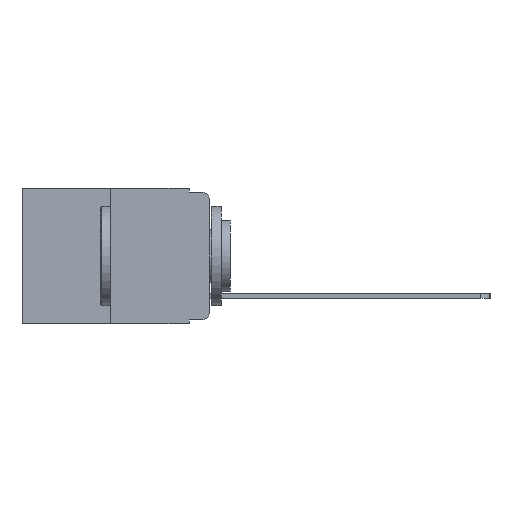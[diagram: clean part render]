
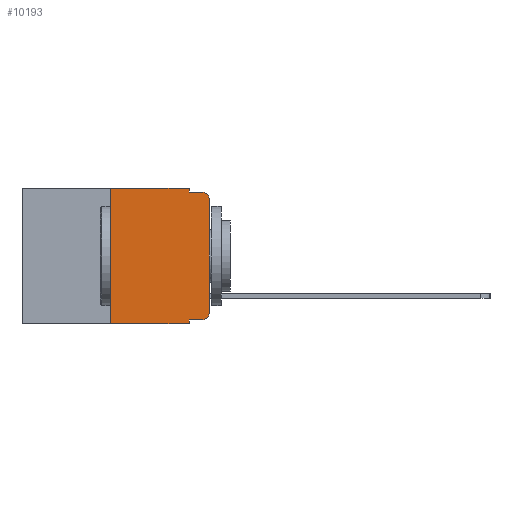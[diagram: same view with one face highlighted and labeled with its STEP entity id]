
A CAD part, left-side view. The second image highlights one B-rep face of the part: STEP entity #10193.
In plain terms, the highlighted planar face has unit normal (-1, 0, 0).
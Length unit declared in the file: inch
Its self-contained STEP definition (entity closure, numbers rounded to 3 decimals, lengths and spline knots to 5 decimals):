
#89 = ORIENTED_EDGE ( 'NONE', *, *, #8027, .F. ) ;
#531 = CARTESIAN_POINT ( 'NONE',  ( 0., 0.051, 0. ) ) ;
#598 = CARTESIAN_POINT ( 'NONE',  ( 0., 0.02, -0.313 ) ) ;
#907 = DIRECTION ( 'NONE',  ( -1., 0., 0. ) ) ;
#2142 = CARTESIAN_POINT ( 'NONE',  ( 0., 0.25, -0.343 ) ) ;
#2165 = LINE ( 'NONE', #4714, #6062 ) ;
#2266 = DIRECTION ( 'NONE',  ( 0., 0., -1. ) ) ;
#2334 = PLANE ( 'NONE',  #13816 ) ;
#2394 = VERTEX_POINT ( 'NONE', #8580 ) ;
#2579 = EDGE_CURVE ( 'NONE', #20101, #2394, #11732, .T. ) ;
#2890 = VECTOR ( 'NONE', #3605, 39.37008 ) ;
#3300 = VECTOR ( 'NONE', #14741, 39.37008 ) ;
#3605 = DIRECTION ( 'NONE',  ( 0., 0., 1. ) ) ;
#3825 = ORIENTED_EDGE ( 'NONE', *, *, #9303, .T. ) ;
#3984 = CARTESIAN_POINT ( 'NONE',  ( 0., 0.473, 0. ) ) ;
#3988 = DIRECTION ( 'NONE',  ( 0., -1., 0. ) ) ;
#3998 = DIRECTION ( 'NONE',  ( 0., 0., 1. ) ) ;
#4028 = CARTESIAN_POINT ( 'NONE',  ( 0., 0., 0. ) ) ;
#4349 = EDGE_CURVE ( 'NONE', #21163, #10808, #13995, .T. ) ;
#4439 = VECTOR ( 'NONE', #20440, 39.37008 ) ;
#4528 = DIRECTION ( 'NONE',  ( 0., -1., 0. ) ) ;
#4602 = CARTESIAN_POINT ( 'NONE',  ( 0., 0.02, -0.333 ) ) ;
#4701 = CARTESIAN_POINT ( 'NONE',  ( 0., 0., -0.03 ) ) ;
#4714 = CARTESIAN_POINT ( 'NONE',  ( 0., 0.473, -0.343 ) ) ;
#4720 = ORIENTED_EDGE ( 'NONE', *, *, #2579, .F. ) ;
#4852 = CARTESIAN_POINT ( 'NONE',  ( 0., 0.473, 0. ) ) ;
#4913 = VECTOR ( 'NONE', #3998, 39.37008 ) ;
#5105 = AXIS2_PLACEMENT_3D ( 'NONE', #598, #12107, #2266 ) ;
#5273 = CARTESIAN_POINT ( 'NONE',  ( 0., 0.25, 0. ) ) ;
#5487 = ORIENTED_EDGE ( 'NONE', *, *, #19863, .F. ) ;
#5658 = DIRECTION ( 'NONE',  ( 0., 0., -1. ) ) ;
#5970 = CIRCLE ( 'NONE', #10265, 0.02 ) ;
#6062 = VECTOR ( 'NONE', #21252, 39.37008 ) ;
#6257 = EDGE_CURVE ( 'NONE', #10003, #12196, #18077, .T. ) ;
#6425 = VERTEX_POINT ( 'NONE', #2142 ) ;
#6624 = EDGE_CURVE ( 'NONE', #12196, #10808, #5970, .T. ) ;
#6947 = VERTEX_POINT ( 'NONE', #4602 ) ;
#7085 = EDGE_LOOP ( 'NONE', ( #21006, #7484, #9443, #5487, #10631, #89, #20883, #4720, #18864, #3825 ) ) ;
#7484 = ORIENTED_EDGE ( 'NONE', *, *, #6624, .T. ) ;
#8027 = EDGE_CURVE ( 'NONE', #6425, #20708, #11605, .T. ) ;
#8580 = CARTESIAN_POINT ( 'NONE',  ( 0., 0.051, -0.343 ) ) ;
#8856 = CARTESIAN_POINT ( 'NONE',  ( 0., 0.051, 0. ) ) ;
#8939 = CARTESIAN_POINT ( 'NONE',  ( 0., 0.051, -0.333 ) ) ;
#9303 = EDGE_CURVE ( 'NONE', #6947, #10003, #19857, .T. ) ;
#9443 = ORIENTED_EDGE ( 'NONE', *, *, #4349, .F. ) ;
#9582 = VECTOR ( 'NONE', #4528, 39.37008 ) ;
#10003 = VERTEX_POINT ( 'NONE', #18994 ) ;
#10193 = ADVANCED_FACE ( 'NONE', ( #15419 ), #2334, .F. ) ;
#10265 = AXIS2_PLACEMENT_3D ( 'NONE', #20912, #907, #18419 ) ;
#10631 = ORIENTED_EDGE ( 'NONE', *, *, #13987, .F. ) ;
#10808 = VERTEX_POINT ( 'NONE', #19141 ) ;
#11506 = LINE ( 'NONE', #4852, #3300 ) ;
#11605 = LINE ( 'NONE', #5273, #2890 ) ;
#11732 = LINE ( 'NONE', #531, #16182 ) ;
#11941 = EDGE_CURVE ( 'NONE', #20101, #6947, #20548, .T. ) ;
#12107 = DIRECTION ( 'NONE',  ( -1., 0., 0. ) ) ;
#12196 = VERTEX_POINT ( 'NONE', #4701 ) ;
#13816 = AXIS2_PLACEMENT_3D ( 'NONE', #3984, #15544, #5658 ) ;
#13987 = EDGE_CURVE ( 'NONE', #20708, #14895, #11506, .T. ) ;
#13995 = LINE ( 'NONE', #14577, #9582 ) ;
#14577 = CARTESIAN_POINT ( 'NONE',  ( 0., 0.051, -0.01 ) ) ;
#14741 = DIRECTION ( 'NONE',  ( 0., -1., 0. ) ) ;
#14895 = VERTEX_POINT ( 'NONE', #20453 ) ;
#15419 = FACE_OUTER_BOUND ( 'NONE', #7085, .T. ) ;
#15544 = DIRECTION ( 'NONE',  ( 1., 0., 0. ) ) ;
#16167 = VECTOR ( 'NONE', #3988, 39.37008 ) ;
#16182 = VECTOR ( 'NONE', #18369, 39.37008 ) ;
#16317 = EDGE_CURVE ( 'NONE', #6425, #2394, #2165, .T. ) ;
#17075 = LINE ( 'NONE', #8856, #4439 ) ;
#17759 = CARTESIAN_POINT ( 'NONE',  ( 0., 0.051, -0.333 ) ) ;
#18077 = LINE ( 'NONE', #4028, #4913 ) ;
#18369 = DIRECTION ( 'NONE',  ( 0., 0., -1. ) ) ;
#18419 = DIRECTION ( 'NONE',  ( 0., 0., -1. ) ) ;
#18864 = ORIENTED_EDGE ( 'NONE', *, *, #11941, .T. ) ;
#18994 = CARTESIAN_POINT ( 'NONE',  ( 0., 0., -0.313 ) ) ;
#19141 = CARTESIAN_POINT ( 'NONE',  ( 0., 0.02, -0.01 ) ) ;
#19857 = CIRCLE ( 'NONE', #5105, 0.02 ) ;
#19863 = EDGE_CURVE ( 'NONE', #14895, #21163, #17075, .T. ) ;
#19869 = CARTESIAN_POINT ( 'NONE',  ( 0., 0.25, 0. ) ) ;
#20101 = VERTEX_POINT ( 'NONE', #17759 ) ;
#20440 = DIRECTION ( 'NONE',  ( 0., 0., -1. ) ) ;
#20453 = CARTESIAN_POINT ( 'NONE',  ( 0., 0.051, 0. ) ) ;
#20548 = LINE ( 'NONE', #8939, #16167 ) ;
#20708 = VERTEX_POINT ( 'NONE', #19869 ) ;
#20883 = ORIENTED_EDGE ( 'NONE', *, *, #16317, .T. ) ;
#20912 = CARTESIAN_POINT ( 'NONE',  ( 0., 0.02, -0.03 ) ) ;
#21006 = ORIENTED_EDGE ( 'NONE', *, *, #6257, .T. ) ;
#21022 = CARTESIAN_POINT ( 'NONE',  ( 0., 0.051, -0.01 ) ) ;
#21163 = VERTEX_POINT ( 'NONE', #21022 ) ;
#21252 = DIRECTION ( 'NONE',  ( 0., -1., 0. ) ) ;
